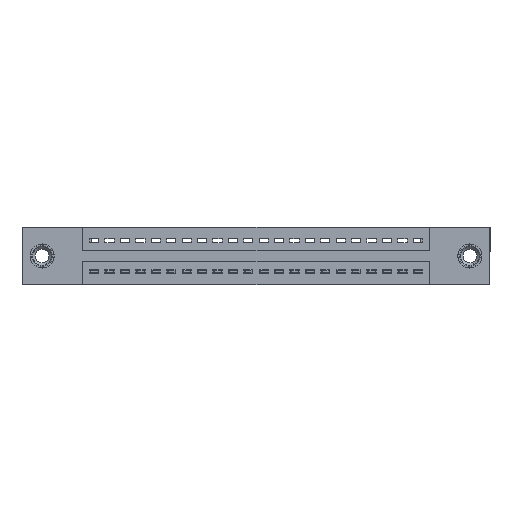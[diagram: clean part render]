
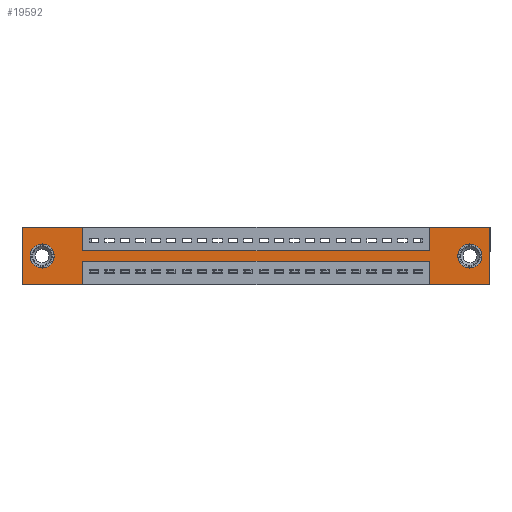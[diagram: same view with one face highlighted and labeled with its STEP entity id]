
A CAD part, front view. The second image highlights one B-rep face of the part: STEP entity #19592.
In plain terms, the highlighted planar face has unit normal (0, -1, 0).
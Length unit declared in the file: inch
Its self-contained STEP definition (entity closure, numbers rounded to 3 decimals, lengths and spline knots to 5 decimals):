
#55 = CARTESIAN_POINT ( 'NONE',  ( 2.6425, 0., 0. ) ) ;
#224 = DIRECTION ( 'NONE',  ( 0., 0., 1. ) ) ;
#408 = VECTOR ( 'NONE', #19836, 39.37008 ) ;
#496 = CARTESIAN_POINT ( 'NONE',  ( 0., 0., 0. ) ) ;
#785 = VECTOR ( 'NONE', #6932, 39.37008 ) ;
#842 = DIRECTION ( 'NONE',  ( 0., 0., 1. ) ) ;
#960 = AXIS2_PLACEMENT_3D ( 'NONE', #1383, #14577, #224 ) ;
#1107 = CARTESIAN_POINT ( 'NONE',  ( 0., 0., 0. ) ) ;
#1139 = CARTESIAN_POINT ( 'NONE',  ( 3.035, 0., 0. ) ) ;
#1383 = CARTESIAN_POINT ( 'NONE',  ( 0.13, 0., -0.185 ) ) ;
#1400 = EDGE_CURVE ( 'NONE', #13155, #8108, #1881, .T. ) ;
#1450 = PLANE ( 'NONE',  #18913 ) ;
#1462 = EDGE_CURVE ( 'NONE', #10531, #10481, #20892, .T. ) ;
#1503 = CARTESIAN_POINT ( 'NONE',  ( 0.13, 0., -0.107 ) ) ;
#1524 = CARTESIAN_POINT ( 'NONE',  ( 2.905, 0., -0.185 ) ) ;
#1598 = CARTESIAN_POINT ( 'NONE',  ( 0.13, 0., -0.185 ) ) ;
#1881 = LINE ( 'NONE', #496, #20138 ) ;
#1908 = LINE ( 'NONE', #5988, #15557 ) ;
#1926 = ORIENTED_EDGE ( 'NONE', *, *, #8734, .F. ) ;
#1964 = VERTEX_POINT ( 'NONE', #15184 ) ;
#2551 = CARTESIAN_POINT ( 'NONE',  ( 2.6425, 0., -0.37 ) ) ;
#2620 = DIRECTION ( 'NONE',  ( 0., 0., -1. ) ) ;
#2748 = EDGE_CURVE ( 'NONE', #13862, #10768, #11309, .T. ) ;
#2865 = DIRECTION ( 'NONE',  ( 0., 0., -1. ) ) ;
#2894 = EDGE_LOOP ( 'NONE', ( #9933, #8527, #14102, #3060, #6734, #5438, #20378, #6964, #16763, #1926, #14371, #7552 ) ) ;
#3029 = DIRECTION ( 'NONE',  ( -1., 0., 0. ) ) ;
#3060 = ORIENTED_EDGE ( 'NONE', *, *, #18721, .F. ) ;
#3108 = CARTESIAN_POINT ( 'NONE',  ( 2.6425, 0., -0.15 ) ) ;
#3580 = CARTESIAN_POINT ( 'NONE',  ( 0., 0., -0.37 ) ) ;
#3724 = DIRECTION ( 'NONE',  ( 1., 0., 0. ) ) ;
#4153 = CARTESIAN_POINT ( 'NONE',  ( 0.3925, 0., -0.22 ) ) ;
#4256 = VERTEX_POINT ( 'NONE', #5355 ) ;
#4390 = CARTESIAN_POINT ( 'NONE',  ( 2.905, 0., -0.107 ) ) ;
#4392 = DIRECTION ( 'NONE',  ( 0., 1., 0. ) ) ;
#4430 = VECTOR ( 'NONE', #8619, 39.37008 ) ;
#4484 = VERTEX_POINT ( 'NONE', #15462 ) ;
#4999 = VERTEX_POINT ( 'NONE', #2551 ) ;
#5131 = VERTEX_POINT ( 'NONE', #3108 ) ;
#5151 = DIRECTION ( 'NONE',  ( 1., 0., 0. ) ) ;
#5218 = LINE ( 'NONE', #3580, #408 ) ;
#5355 = CARTESIAN_POINT ( 'NONE',  ( 0.3925, 0., 0. ) ) ;
#5438 = ORIENTED_EDGE ( 'NONE', *, *, #9204, .F. ) ;
#5503 = DIRECTION ( 'NONE',  ( -1., 0., 0. ) ) ;
#5669 = CARTESIAN_POINT ( 'NONE',  ( 0., 0., -0.37 ) ) ;
#5955 = EDGE_CURVE ( 'NONE', #4999, #1964, #12140, .T. ) ;
#5988 = CARTESIAN_POINT ( 'NONE',  ( 0.3925, 0., -0.37 ) ) ;
#6153 = LINE ( 'NONE', #9638, #15731 ) ;
#6211 = EDGE_CURVE ( 'NONE', #5131, #12740, #19606, .T. ) ;
#6325 = CARTESIAN_POINT ( 'NONE',  ( 2.905, 0., -0.263 ) ) ;
#6355 = VECTOR ( 'NONE', #9241, 39.37008 ) ;
#6403 = ORIENTED_EDGE ( 'NONE', *, *, #2748, .T. ) ;
#6437 = DIRECTION ( 'NONE',  ( 0., 0., -1. ) ) ;
#6548 = CARTESIAN_POINT ( 'NONE',  ( 0., 0., 0. ) ) ;
#6626 = CARTESIAN_POINT ( 'NONE',  ( 0.13, 0., -0.263 ) ) ;
#6713 = ORIENTED_EDGE ( 'NONE', *, *, #1462, .T. ) ;
#6734 = ORIENTED_EDGE ( 'NONE', *, *, #7597, .F. ) ;
#6817 = AXIS2_PLACEMENT_3D ( 'NONE', #20933, #4392, #14473 ) ;
#6932 = DIRECTION ( 'NONE',  ( 0., 0., -1. ) ) ;
#6949 = CARTESIAN_POINT ( 'NONE',  ( 0., 0., 0. ) ) ;
#6964 = ORIENTED_EDGE ( 'NONE', *, *, #16944, .F. ) ;
#7425 = VECTOR ( 'NONE', #2620, 39.37008 ) ;
#7552 = ORIENTED_EDGE ( 'NONE', *, *, #12366, .F. ) ;
#7597 = EDGE_CURVE ( 'NONE', #9555, #4484, #8656, .T. ) ;
#7691 = EDGE_CURVE ( 'NONE', #10481, #10531, #16215, .T. ) ;
#7817 = AXIS2_PLACEMENT_3D ( 'NONE', #1524, #14584, #6437 ) ;
#8108 = VERTEX_POINT ( 'NONE', #6548 ) ;
#8527 = ORIENTED_EDGE ( 'NONE', *, *, #18777, .F. ) ;
#8599 = CARTESIAN_POINT ( 'NONE',  ( 0.3925, 0., 0. ) ) ;
#8619 = DIRECTION ( 'NONE',  ( 0., 0., 1. ) ) ;
#8656 = LINE ( 'NONE', #1139, #7425 ) ;
#8716 = FACE_OUTER_BOUND ( 'NONE', #2894, .T. ) ;
#8734 = EDGE_CURVE ( 'NONE', #8108, #4256, #18242, .T. ) ;
#8908 = VECTOR ( 'NONE', #3029, 39.37008 ) ;
#9204 = EDGE_CURVE ( 'NONE', #12740, #9555, #10976, .T. ) ;
#9241 = DIRECTION ( 'NONE',  ( 1., 0., 0. ) ) ;
#9555 = VERTEX_POINT ( 'NONE', #12329 ) ;
#9638 = CARTESIAN_POINT ( 'NONE',  ( 0.3925, 0., -0.15 ) ) ;
#9837 = DIRECTION ( 'NONE',  ( 0., 0., -1. ) ) ;
#9933 = ORIENTED_EDGE ( 'NONE', *, *, #11845, .F. ) ;
#10481 = VERTEX_POINT ( 'NONE', #1503 ) ;
#10531 = VERTEX_POINT ( 'NONE', #6626 ) ;
#10768 = VERTEX_POINT ( 'NONE', #6325 ) ;
#10872 = VECTOR ( 'NONE', #5503, 39.37008 ) ;
#10976 = LINE ( 'NONE', #1107, #6355 ) ;
#11085 = FACE_BOUND ( 'NONE', #11259, .T. ) ;
#11259 = EDGE_LOOP ( 'NONE', ( #15742, #6713 ) ) ;
#11309 = CIRCLE ( 'NONE', #6817, 0.078 ) ;
#11845 = EDGE_CURVE ( 'NONE', #14880, #15948, #1908, .T. ) ;
#12140 = LINE ( 'NONE', #15256, #4430 ) ;
#12329 = CARTESIAN_POINT ( 'NONE',  ( 3.035, 0., 0. ) ) ;
#12366 = EDGE_CURVE ( 'NONE', #15948, #13155, #16677, .T. ) ;
#12740 = VERTEX_POINT ( 'NONE', #55 ) ;
#12901 = VECTOR ( 'NONE', #842, 39.37008 ) ;
#13155 = VERTEX_POINT ( 'NONE', #5669 ) ;
#13193 = DIRECTION ( 'NONE',  ( 0., -1., 0. ) ) ;
#13339 = ORIENTED_EDGE ( 'NONE', *, *, #20923, .T. ) ;
#13577 = VERTEX_POINT ( 'NONE', #18542 ) ;
#13579 = DIRECTION ( 'NONE',  ( 0., 0., 1. ) ) ;
#13740 = CARTESIAN_POINT ( 'NONE',  ( 0.3925, 0., -0.37 ) ) ;
#13862 = VERTEX_POINT ( 'NONE', #4390 ) ;
#14102 = ORIENTED_EDGE ( 'NONE', *, *, #5955, .F. ) ;
#14211 = EDGE_LOOP ( 'NONE', ( #6403, #13339 ) ) ;
#14371 = ORIENTED_EDGE ( 'NONE', *, *, #1400, .F. ) ;
#14381 = CIRCLE ( 'NONE', #7817, 0.078 ) ;
#14473 = DIRECTION ( 'NONE',  ( 0., 0., -1. ) ) ;
#14577 = DIRECTION ( 'NONE',  ( 0., 1., 0. ) ) ;
#14584 = DIRECTION ( 'NONE',  ( 0., 1., 0. ) ) ;
#14724 = DIRECTION ( 'NONE',  ( 0., 1., 0. ) ) ;
#14867 = LINE ( 'NONE', #8599, #785 ) ;
#14880 = VERTEX_POINT ( 'NONE', #4153 ) ;
#15184 = CARTESIAN_POINT ( 'NONE',  ( 2.6425, 0., -0.22 ) ) ;
#15256 = CARTESIAN_POINT ( 'NONE',  ( 2.6425, 0., -0.37 ) ) ;
#15286 = LINE ( 'NONE', #17105, #10872 ) ;
#15445 = VECTOR ( 'NONE', #3724, 39.37008 ) ;
#15462 = CARTESIAN_POINT ( 'NONE',  ( 3.035, 0., -0.37 ) ) ;
#15477 = CARTESIAN_POINT ( 'NONE',  ( 2.6425, 0., 0. ) ) ;
#15557 = VECTOR ( 'NONE', #2865, 39.37008 ) ;
#15731 = VECTOR ( 'NONE', #5151, 39.37008 ) ;
#15742 = ORIENTED_EDGE ( 'NONE', *, *, #7691, .T. ) ;
#15948 = VERTEX_POINT ( 'NONE', #13740 ) ;
#16215 = CIRCLE ( 'NONE', #21206, 0.078 ) ;
#16370 = DIRECTION ( 'NONE',  ( 0., 0., 1. ) ) ;
#16677 = LINE ( 'NONE', #16712, #8908 ) ;
#16712 = CARTESIAN_POINT ( 'NONE',  ( 0., 0., -0.37 ) ) ;
#16763 = ORIENTED_EDGE ( 'NONE', *, *, #17771, .F. ) ;
#16944 = EDGE_CURVE ( 'NONE', #13577, #5131, #6153, .T. ) ;
#17105 = CARTESIAN_POINT ( 'NONE',  ( 0.3925, 0., -0.22 ) ) ;
#17771 = EDGE_CURVE ( 'NONE', #4256, #13577, #14867, .T. ) ;
#17885 = CARTESIAN_POINT ( 'NONE',  ( 0., 0., -0.37 ) ) ;
#18242 = LINE ( 'NONE', #6949, #15445 ) ;
#18542 = CARTESIAN_POINT ( 'NONE',  ( 0.3925, 0., -0.15 ) ) ;
#18721 = EDGE_CURVE ( 'NONE', #4484, #4999, #5218, .T. ) ;
#18777 = EDGE_CURVE ( 'NONE', #1964, #14880, #15286, .T. ) ;
#18913 = AXIS2_PLACEMENT_3D ( 'NONE', #17885, #13193, #9837 ) ;
#19592 = ADVANCED_FACE ( 'NONE', ( #20368, #11085, #8716 ), #1450, .T. ) ;
#19606 = LINE ( 'NONE', #15477, #12901 ) ;
#19836 = DIRECTION ( 'NONE',  ( -1., 0., 0. ) ) ;
#20138 = VECTOR ( 'NONE', #13579, 39.37008 ) ;
#20368 = FACE_BOUND ( 'NONE', #14211, .T. ) ;
#20378 = ORIENTED_EDGE ( 'NONE', *, *, #6211, .F. ) ;
#20892 = CIRCLE ( 'NONE', #960, 0.078 ) ;
#20923 = EDGE_CURVE ( 'NONE', #10768, #13862, #14381, .T. ) ;
#20933 = CARTESIAN_POINT ( 'NONE',  ( 2.905, 0., -0.185 ) ) ;
#21206 = AXIS2_PLACEMENT_3D ( 'NONE', #1598, #14724, #16370 ) ;
